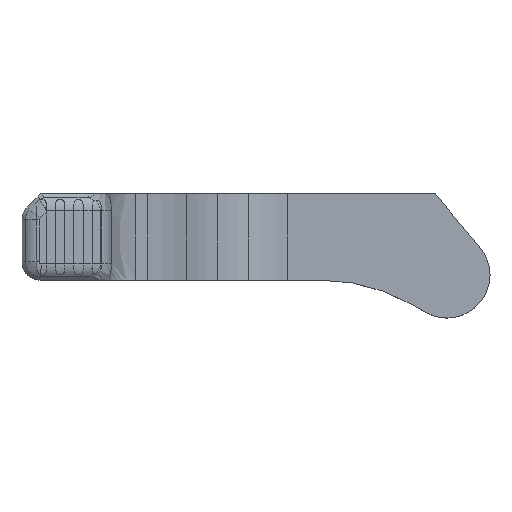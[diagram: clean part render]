
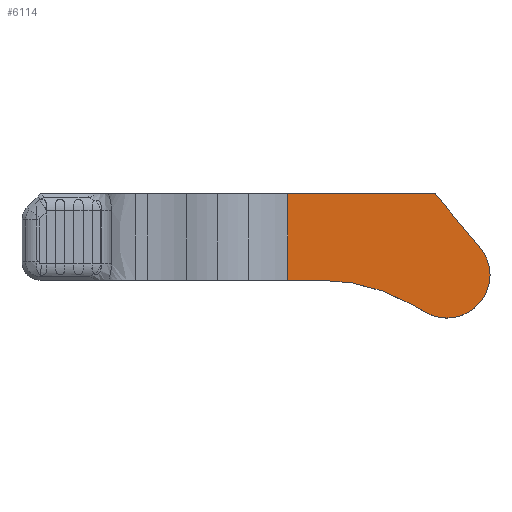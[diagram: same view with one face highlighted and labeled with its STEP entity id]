
A CAD part, top view. The second image highlights one B-rep face of the part: STEP entity #6114.
In plain terms, the highlighted planar face has unit normal (0, 0, 1).
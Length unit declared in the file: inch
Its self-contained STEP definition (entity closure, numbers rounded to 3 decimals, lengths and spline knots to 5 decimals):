
#102 = DIRECTION ( 'NONE',  ( -0.643, 0.766, 0. ) ) ;
#117 = VERTEX_POINT ( 'NONE', #3442 ) ;
#187 = VECTOR ( 'NONE', #3651, 39.37008 ) ;
#316 = CARTESIAN_POINT ( 'NONE',  ( -2.2157, 0.4418, 0.2 ) ) ;
#466 = CARTESIAN_POINT ( 'NONE',  ( -0.1175, -0.20352, 0.2 ) ) ;
#646 = DIRECTION ( 'NONE',  ( 0., 0., 1. ) ) ;
#860 = VERTEX_POINT ( 'NONE', #9621 ) ;
#1151 = ORIENTED_EDGE ( 'NONE', *, *, #11838, .T. ) ;
#1227 = DIRECTION ( 'NONE',  ( -1., 0., 0. ) ) ;
#2208 = ORIENTED_EDGE ( 'NONE', *, *, #8989, .T. ) ;
#2235 = LINE ( 'NONE', #5921, #8245 ) ;
#2452 = EDGE_CURVE ( 'NONE', #117, #6120, #7546, .T. ) ;
#2612 = EDGE_CURVE ( 'NONE', #10394, #860, #9318, .T. ) ;
#3030 = CARTESIAN_POINT ( 'NONE',  ( 0.18002, 0.15106, 0.2 ) ) ;
#3442 = CARTESIAN_POINT ( 'NONE',  ( -0.06394, 0.4418, 0.2 ) ) ;
#3528 = CARTESIAN_POINT ( 'NONE',  ( 0., 0., 0.2 ) ) ;
#3599 = ORIENTED_EDGE ( 'NONE', *, *, #4522, .T. ) ;
#3651 = DIRECTION ( 'NONE',  ( 0., -1., 0. ) ) ;
#3746 = VECTOR ( 'NONE', #4157, 39.37008 ) ;
#3897 = AXIS2_PLACEMENT_3D ( 'NONE', #3528, #646, #7395 ) ;
#4102 = EDGE_CURVE ( 'NONE', #10702, #117, #5677, .T. ) ;
#4157 = DIRECTION ( 'NONE',  ( 0.866, -0.5, 0. ) ) ;
#4458 = EDGE_CURVE ( 'NONE', #8909, #10702, #9188, .T. ) ;
#4522 = EDGE_CURVE ( 'NONE', #6120, #8710, #10047, .T. ) ;
#4721 = DIRECTION ( 'NONE',  ( 0., 0., -1. ) ) ;
#4842 = DIRECTION ( 'NONE',  ( -1., 0., 0. ) ) ;
#5096 = AXIS2_PLACEMENT_3D ( 'NONE', #5710, #4721, #6816 ) ;
#5399 = ORIENTED_EDGE ( 'NONE', *, *, #4458, .T. ) ;
#5677 = LINE ( 'NONE', #8509, #10173 ) ;
#5710 = CARTESIAN_POINT ( 'NONE',  ( -0.68911, -1.0282, 0.2 ) ) ;
#5921 = CARTESIAN_POINT ( 'NONE',  ( -0.68911, -0.0282, 0.2 ) ) ;
#6087 = ORIENTED_EDGE ( 'NONE', *, *, #4102, .T. ) ;
#6114 = ADVANCED_FACE ( 'NONE', ( #8605 ), #11326, .F. ) ;
#6120 = VERTEX_POINT ( 'NONE', #10582 ) ;
#6816 = DIRECTION ( 'NONE',  ( -1., 0., 0. ) ) ;
#6922 = CARTESIAN_POINT ( 'NONE',  ( -0.68911, -0.0282, 0.2 ) ) ;
#7395 = DIRECTION ( 'NONE',  ( 1., 0., 0. ) ) ;
#7546 = LINE ( 'NONE', #316, #8930 ) ;
#7658 = LINE ( 'NONE', #7904, #3746 ) ;
#7904 = CARTESIAN_POINT ( 'NONE',  ( -0.1175, -0.20352, 0.2 ) ) ;
#8124 = AXIS2_PLACEMENT_3D ( 'NONE', #11508, #8477, #1227 ) ;
#8245 = VECTOR ( 'NONE', #8809, 39.37008 ) ;
#8389 = CARTESIAN_POINT ( 'NONE',  ( -0.86627, -0.0282, 0.2 ) ) ;
#8477 = DIRECTION ( 'NONE',  ( 0., 0., -1. ) ) ;
#8509 = CARTESIAN_POINT ( 'NONE',  ( -0.06394, 0.4418, 0.2 ) ) ;
#8605 = FACE_OUTER_BOUND ( 'NONE', #11627, .T. ) ;
#8710 = VERTEX_POINT ( 'NONE', #8389 ) ;
#8809 = DIRECTION ( 'NONE',  ( 1., 0., 0. ) ) ;
#8909 = VERTEX_POINT ( 'NONE', #466 ) ;
#8930 = VECTOR ( 'NONE', #4842, 39.37008 ) ;
#8989 = EDGE_CURVE ( 'NONE', #8710, #10394, #2235, .T. ) ;
#9188 = CIRCLE ( 'NONE', #3897, 0.235 ) ;
#9318 = CIRCLE ( 'NONE', #8124, 1. ) ;
#9621 = CARTESIAN_POINT ( 'NONE',  ( -0.18911, -0.16217, 0.2 ) ) ;
#10047 = LINE ( 'NONE', #10984, #187 ) ;
#10173 = VECTOR ( 'NONE', #102, 39.37008 ) ;
#10394 = VERTEX_POINT ( 'NONE', #6922 ) ;
#10582 = CARTESIAN_POINT ( 'NONE',  ( -0.86627, 0.4418, 0.2 ) ) ;
#10702 = VERTEX_POINT ( 'NONE', #3030 ) ;
#10879 = ORIENTED_EDGE ( 'NONE', *, *, #2612, .T. ) ;
#10984 = CARTESIAN_POINT ( 'NONE',  ( -0.86627, -1.0282, 0.2 ) ) ;
#11274 = ORIENTED_EDGE ( 'NONE', *, *, #2452, .T. ) ;
#11326 = PLANE ( 'NONE',  #5096 ) ;
#11508 = CARTESIAN_POINT ( 'NONE',  ( -0.68911, -1.0282, 0.2 ) ) ;
#11627 = EDGE_LOOP ( 'NONE', ( #11274, #3599, #2208, #10879, #1151, #5399, #6087 ) ) ;
#11838 = EDGE_CURVE ( 'NONE', #860, #8909, #7658, .T. ) ;
